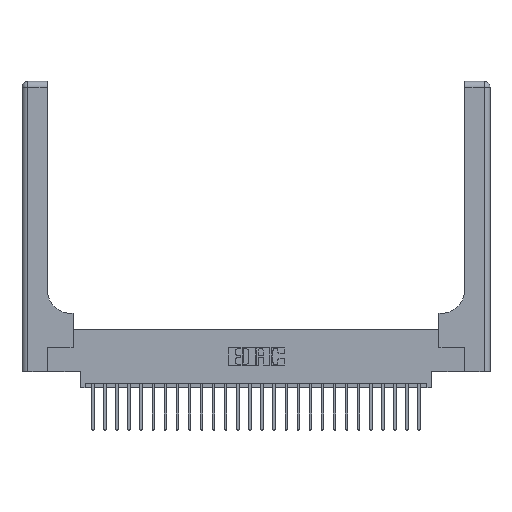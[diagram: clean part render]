
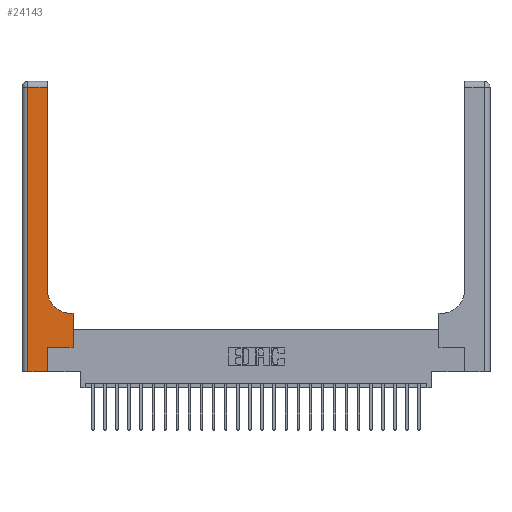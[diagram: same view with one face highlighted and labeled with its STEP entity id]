
A CAD part, top view. The second image highlights one B-rep face of the part: STEP entity #24143.
In plain terms, the highlighted planar face has unit normal (0, 0, 1).
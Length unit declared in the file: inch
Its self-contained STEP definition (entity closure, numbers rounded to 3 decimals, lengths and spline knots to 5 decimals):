
#221 = CARTESIAN_POINT ( 'NONE',  ( 0.265, 0.25, 0.37 ) ) ;
#344 = VERTEX_POINT ( 'NONE', #221 ) ;
#673 = VERTEX_POINT ( 'NONE', #2754 ) ;
#764 = DIRECTION ( 'NONE',  ( -1., 0., 0. ) ) ;
#1038 = FACE_OUTER_BOUND ( 'NONE', #17136, .T. ) ;
#1362 = VECTOR ( 'NONE', #11226, 39.37008 ) ;
#1578 = VERTEX_POINT ( 'NONE', #19280 ) ;
#1749 = DIRECTION ( 'NONE',  ( -1., 0., 0. ) ) ;
#2042 = VERTEX_POINT ( 'NONE', #22858 ) ;
#2153 = CARTESIAN_POINT ( 'NONE',  ( 0.265, 0.25, 0.37 ) ) ;
#2428 = EDGE_CURVE ( 'NONE', #344, #2042, #13883, .T. ) ;
#2754 = CARTESIAN_POINT ( 'NONE',  ( 0.26, 2.94, 0.37 ) ) ;
#2933 = CARTESIAN_POINT ( 'NONE',  ( 0.06, 3., 0.37 ) ) ;
#3238 = ORIENTED_EDGE ( 'NONE', *, *, #15707, .T. ) ;
#3360 = EDGE_CURVE ( 'NONE', #673, #13140, #13213, .T. ) ;
#4915 = DIRECTION ( 'NONE',  ( 0., -1., 0. ) ) ;
#5117 = DIRECTION ( 'NONE',  ( -1., 0., 0. ) ) ;
#5364 = EDGE_CURVE ( 'NONE', #1578, #344, #7236, .T. ) ;
#5417 = ORIENTED_EDGE ( 'NONE', *, *, #13230, .T. ) ;
#5930 = VECTOR ( 'NONE', #15043, 39.37008 ) ;
#6045 = ORIENTED_EDGE ( 'NONE', *, *, #15247, .T. ) ;
#6812 = EDGE_CURVE ( 'NONE', #2042, #24431, #16421, .T. ) ;
#7236 = LINE ( 'NONE', #7249, #1362 ) ;
#7249 = CARTESIAN_POINT ( 'NONE',  ( 0.265, 0., 0.37 ) ) ;
#7432 = AXIS2_PLACEMENT_3D ( 'NONE', #20111, #8278, #22100 ) ;
#8278 = DIRECTION ( 'NONE',  ( 0., 0., -1. ) ) ;
#9583 = DIRECTION ( 'NONE',  ( 1., 0., 0. ) ) ;
#10307 = VECTOR ( 'NONE', #4915, 39.37008 ) ;
#10341 = ORIENTED_EDGE ( 'NONE', *, *, #3360, .T. ) ;
#10635 = CARTESIAN_POINT ( 'NONE',  ( 0., 2.94, 0.37 ) ) ;
#11226 = DIRECTION ( 'NONE',  ( 0., 1., 0. ) ) ;
#11598 = CARTESIAN_POINT ( 'NONE',  ( 0.26, 0.6, 0.37 ) ) ;
#11723 = CARTESIAN_POINT ( 'NONE',  ( 0.26, 0.85, 0.37 ) ) ;
#11727 = VECTOR ( 'NONE', #9583, 39.37008 ) ;
#11906 = CIRCLE ( 'NONE', #7432, 0.25 ) ;
#12855 = CARTESIAN_POINT ( 'NONE',  ( 0.06, 0., 0.37 ) ) ;
#12961 = PLANE ( 'NONE',  #21412 ) ;
#13140 = VERTEX_POINT ( 'NONE', #23001 ) ;
#13213 = LINE ( 'NONE', #10635, #23077 ) ;
#13230 = EDGE_CURVE ( 'NONE', #22928, #673, #19717, .T. ) ;
#13607 = VECTOR ( 'NONE', #1749, 39.37008 ) ;
#13728 = CARTESIAN_POINT ( 'NONE',  ( 0.528, 0.6, 0.37 ) ) ;
#13883 = LINE ( 'NONE', #2153, #18503 ) ;
#13960 = ORIENTED_EDGE ( 'NONE', *, *, #24711, .T. ) ;
#14471 = VECTOR ( 'NONE', #23248, 39.37008 ) ;
#15043 = DIRECTION ( 'NONE',  ( 0., 1., 0. ) ) ;
#15247 = EDGE_CURVE ( 'NONE', #24431, #23563, #18864, .T. ) ;
#15335 = CARTESIAN_POINT ( 'NONE',  ( 0.51, 0.6, 0.37 ) ) ;
#15547 = CARTESIAN_POINT ( 'NONE',  ( 0., 0., 0.37 ) ) ;
#15556 = LINE ( 'NONE', #2933, #10307 ) ;
#15707 = EDGE_CURVE ( 'NONE', #22704, #1578, #22231, .T. ) ;
#16421 = LINE ( 'NONE', #22958, #5930 ) ;
#16425 = ORIENTED_EDGE ( 'NONE', *, *, #5364, .T. ) ;
#16919 = DIRECTION ( 'NONE',  ( 0., 0., -1. ) ) ;
#17136 = EDGE_LOOP ( 'NONE', ( #5417, #10341, #13960, #3238, #16425, #19923, #24459, #6045, #18479 ) ) ;
#17929 = DIRECTION ( 'NONE',  ( 1., 0., 0. ) ) ;
#18479 = ORIENTED_EDGE ( 'NONE', *, *, #19173, .T. ) ;
#18503 = VECTOR ( 'NONE', #17929, 39.37008 ) ;
#18864 = LINE ( 'NONE', #11598, #13607 ) ;
#19173 = EDGE_CURVE ( 'NONE', #23563, #22928, #11906, .T. ) ;
#19280 = CARTESIAN_POINT ( 'NONE',  ( 0.265, 0., 0.37 ) ) ;
#19717 = LINE ( 'NONE', #21292, #14471 ) ;
#19923 = ORIENTED_EDGE ( 'NONE', *, *, #2428, .T. ) ;
#20111 = CARTESIAN_POINT ( 'NONE',  ( 0.51, 0.85, 0.37 ) ) ;
#20832 = CARTESIAN_POINT ( 'NONE',  ( 0., 3., 0.37 ) ) ;
#21292 = CARTESIAN_POINT ( 'NONE',  ( 0.26, 3., 0.37 ) ) ;
#21412 = AXIS2_PLACEMENT_3D ( 'NONE', #20832, #16919, #5117 ) ;
#22100 = DIRECTION ( 'NONE',  ( 1., 0., 0. ) ) ;
#22231 = LINE ( 'NONE', #15547, #11727 ) ;
#22704 = VERTEX_POINT ( 'NONE', #12855 ) ;
#22858 = CARTESIAN_POINT ( 'NONE',  ( 0.528, 0.25, 0.37 ) ) ;
#22928 = VERTEX_POINT ( 'NONE', #11723 ) ;
#22958 = CARTESIAN_POINT ( 'NONE',  ( 0.528, 0.25, 0.37 ) ) ;
#23001 = CARTESIAN_POINT ( 'NONE',  ( 0.06, 2.94, 0.37 ) ) ;
#23077 = VECTOR ( 'NONE', #764, 39.37008 ) ;
#23248 = DIRECTION ( 'NONE',  ( 0., 1., 0. ) ) ;
#23563 = VERTEX_POINT ( 'NONE', #15335 ) ;
#24143 = ADVANCED_FACE ( 'NONE', ( #1038 ), #12961, .F. ) ;
#24431 = VERTEX_POINT ( 'NONE', #13728 ) ;
#24459 = ORIENTED_EDGE ( 'NONE', *, *, #6812, .T. ) ;
#24711 = EDGE_CURVE ( 'NONE', #13140, #22704, #15556, .T. ) ;
